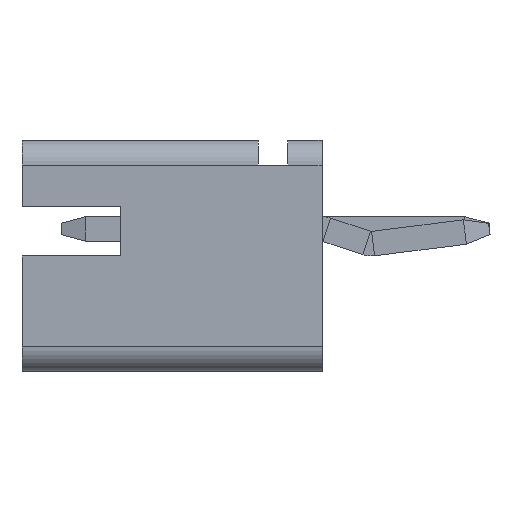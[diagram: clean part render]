
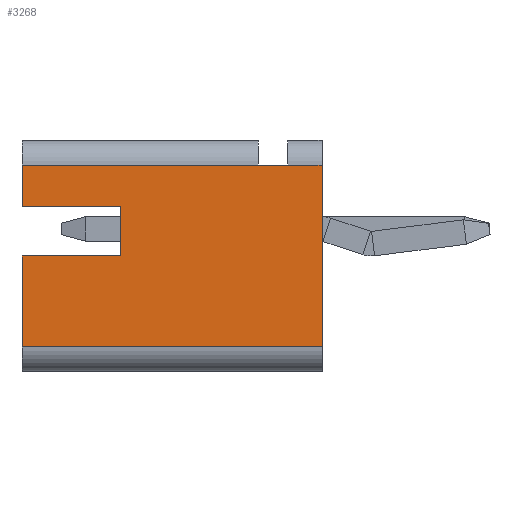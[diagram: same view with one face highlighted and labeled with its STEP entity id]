
A CAD part, left-side view. The second image highlights one B-rep face of the part: STEP entity #3268.
In plain terms, the highlighted planar face has unit normal (-1, 0, 0).
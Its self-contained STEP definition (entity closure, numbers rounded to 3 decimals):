
#137 = CARTESIAN_POINT ( 'NONE',  ( -2., 4.1, 0.45 ) ) ;
#172 = EDGE_CURVE ( 'NONE', #2581, #920, #2140, .T. ) ;
#308 = LINE ( 'NONE', #2070, #589 ) ;
#325 = VERTEX_POINT ( 'NONE', #4972 ) ;
#396 = CARTESIAN_POINT ( 'NONE',  ( -2., 6.1, 1.8 ) ) ;
#403 = CARTESIAN_POINT ( 'NONE',  ( -2., 0., -2.4 ) ) ;
#589 = VECTOR ( 'NONE', #2565, 1000. ) ;
#611 = ORIENTED_EDGE ( 'NONE', *, *, #172, .T. ) ;
#870 = CARTESIAN_POINT ( 'NONE',  ( -2., 6.1, -0.55 ) ) ;
#920 = VERTEX_POINT ( 'NONE', #3400 ) ;
#1004 = VERTEX_POINT ( 'NONE', #3978 ) ;
#1055 = ORIENTED_EDGE ( 'NONE', *, *, #5172, .F. ) ;
#1146 = VERTEX_POINT ( 'NONE', #5788 ) ;
#1151 = FACE_OUTER_BOUND ( 'NONE', #4481, .T. ) ;
#1154 = DIRECTION ( 'NONE',  ( 0., 1., 0. ) ) ;
#1155 = EDGE_CURVE ( 'NONE', #1146, #2173, #3998, .T. ) ;
#1301 = LINE ( 'NONE', #870, #3153 ) ;
#1326 = CARTESIAN_POINT ( 'NONE',  ( -2., 0., 1.8 ) ) ;
#1393 = ORIENTED_EDGE ( 'NONE', *, *, #3509, .F. ) ;
#1527 = LINE ( 'NONE', #2558, #2939 ) ;
#1877 = ORIENTED_EDGE ( 'NONE', *, *, #4105, .F. ) ;
#1885 = ORIENTED_EDGE ( 'NONE', *, *, #1155, .T. ) ;
#1910 = LINE ( 'NONE', #396, #5253 ) ;
#2065 = EDGE_CURVE ( 'NONE', #5258, #4396, #1527, .T. ) ;
#2070 = CARTESIAN_POINT ( 'NONE',  ( -2., 4.1, 0.45 ) ) ;
#2093 = CARTESIAN_POINT ( 'NONE',  ( -2., 6.1, -0.55 ) ) ;
#2140 = LINE ( 'NONE', #4085, #5765 ) ;
#2173 = VERTEX_POINT ( 'NONE', #3155 ) ;
#2205 = DIRECTION ( 'NONE',  ( 0., 0., -1. ) ) ;
#2221 = EDGE_CURVE ( 'NONE', #1146, #920, #5731, .T. ) ;
#2246 = ORIENTED_EDGE ( 'NONE', *, *, #2065, .T. ) ;
#2496 = CARTESIAN_POINT ( 'NONE',  ( -2., 6.1, -2.4 ) ) ;
#2558 = CARTESIAN_POINT ( 'NONE',  ( -2., 0., -2.4 ) ) ;
#2565 = DIRECTION ( 'NONE',  ( 0., 0., 1. ) ) ;
#2581 = VERTEX_POINT ( 'NONE', #3921 ) ;
#2596 = DIRECTION ( 'NONE',  ( 1., 0., 0. ) ) ;
#2725 = VECTOR ( 'NONE', #5322, 1000. ) ;
#2939 = VECTOR ( 'NONE', #3684, 1000. ) ;
#2966 = LINE ( 'NONE', #1326, #5855 ) ;
#3028 = DIRECTION ( 'NONE',  ( 0., 0., -1. ) ) ;
#3031 = CARTESIAN_POINT ( 'NONE',  ( -2., 6.1, -0.55 ) ) ;
#3153 = VECTOR ( 'NONE', #5565, 1000. ) ;
#3155 = CARTESIAN_POINT ( 'NONE',  ( -2., 6.1, 1.3 ) ) ;
#3233 = ORIENTED_EDGE ( 'NONE', *, *, #5393, .F. ) ;
#3268 = ADVANCED_FACE ( 'NONE', ( #1151 ), #5900, .F. ) ;
#3289 = ORIENTED_EDGE ( 'NONE', *, *, #2221, .F. ) ;
#3400 = CARTESIAN_POINT ( 'NONE',  ( -2., 0.7, 1.3 ) ) ;
#3509 = EDGE_CURVE ( 'NONE', #5404, #1004, #1301, .T. ) ;
#3684 = DIRECTION ( 'NONE',  ( 0., -1., 0. ) ) ;
#3757 = AXIS2_PLACEMENT_3D ( 'NONE', #5864, #2596, #3028 ) ;
#3820 = VERTEX_POINT ( 'NONE', #137 ) ;
#3858 = VECTOR ( 'NONE', #4439, 1000. ) ;
#3921 = CARTESIAN_POINT ( 'NONE',  ( -2., 0., 1.3 ) ) ;
#3978 = CARTESIAN_POINT ( 'NONE',  ( -2., 4.1, -0.55 ) ) ;
#3998 = LINE ( 'NONE', #4862, #2725 ) ;
#4085 = CARTESIAN_POINT ( 'NONE',  ( -2., 0., 1.3 ) ) ;
#4105 = EDGE_CURVE ( 'NONE', #2581, #4396, #2966, .T. ) ;
#4188 = DIRECTION ( 'NONE',  ( 0., 0., 1. ) ) ;
#4396 = VERTEX_POINT ( 'NONE', #403 ) ;
#4439 = DIRECTION ( 'NONE',  ( 0., 0., 1. ) ) ;
#4459 = EDGE_CURVE ( 'NONE', #3820, #325, #5772, .T. ) ;
#4481 = EDGE_LOOP ( 'NONE', ( #3233, #2246, #1877, #611, #3289, #1885, #1055, #5503, #4884, #1393 ) ) ;
#4527 = VECTOR ( 'NONE', #5534, 1000. ) ;
#4550 = CARTESIAN_POINT ( 'NONE',  ( -2., 1.3, 1.3 ) ) ;
#4862 = CARTESIAN_POINT ( 'NONE',  ( -2., 0., 1.3 ) ) ;
#4884 = ORIENTED_EDGE ( 'NONE', *, *, #5626, .F. ) ;
#4972 = CARTESIAN_POINT ( 'NONE',  ( -2., 6.1, 0.45 ) ) ;
#5117 = LINE ( 'NONE', #2093, #3858 ) ;
#5172 = EDGE_CURVE ( 'NONE', #325, #2173, #1910, .T. ) ;
#5253 = VECTOR ( 'NONE', #4188, 1000. ) ;
#5258 = VERTEX_POINT ( 'NONE', #2496 ) ;
#5322 = DIRECTION ( 'NONE',  ( 0., 1., 0. ) ) ;
#5369 = VECTOR ( 'NONE', #5544, 1000. ) ;
#5393 = EDGE_CURVE ( 'NONE', #5258, #5404, #5117, .T. ) ;
#5404 = VERTEX_POINT ( 'NONE', #3031 ) ;
#5503 = ORIENTED_EDGE ( 'NONE', *, *, #4459, .F. ) ;
#5534 = DIRECTION ( 'NONE',  ( 0., 1., 0. ) ) ;
#5544 = DIRECTION ( 'NONE',  ( 0., -1., 0. ) ) ;
#5565 = DIRECTION ( 'NONE',  ( 0., -1., 0. ) ) ;
#5626 = EDGE_CURVE ( 'NONE', #1004, #3820, #308, .T. ) ;
#5731 = LINE ( 'NONE', #4550, #5369 ) ;
#5765 = VECTOR ( 'NONE', #1154, 1000. ) ;
#5772 = LINE ( 'NONE', #6036, #4527 ) ;
#5788 = CARTESIAN_POINT ( 'NONE',  ( -2., 1.3, 1.3 ) ) ;
#5855 = VECTOR ( 'NONE', #2205, 1000. ) ;
#5864 = CARTESIAN_POINT ( 'NONE',  ( -2., 0., 0. ) ) ;
#5900 = PLANE ( 'NONE',  #3757 ) ;
#6036 = CARTESIAN_POINT ( 'NONE',  ( -2., 6.1, 0.45 ) ) ;
